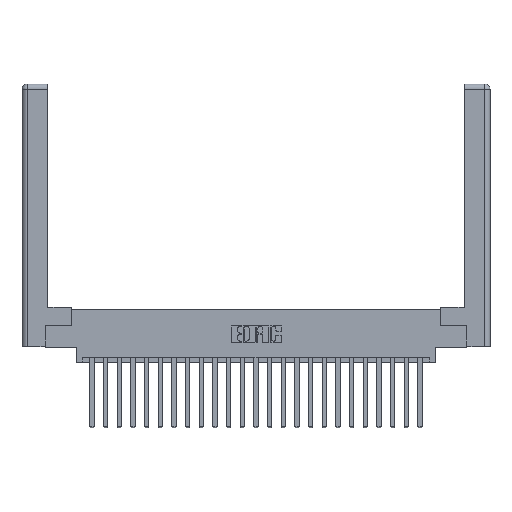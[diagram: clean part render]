
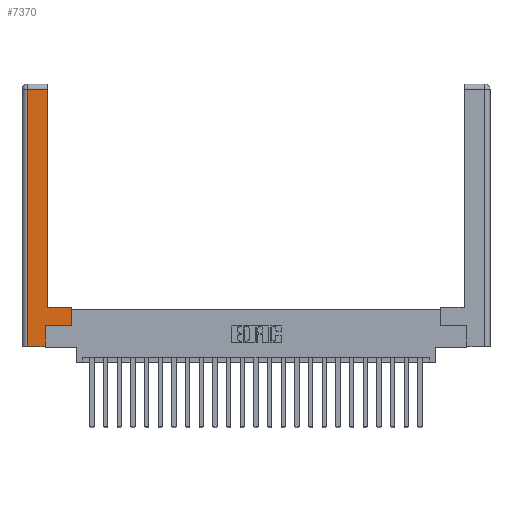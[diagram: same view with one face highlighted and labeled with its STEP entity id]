
A CAD part, top view. The second image highlights one B-rep face of the part: STEP entity #7370.
In plain terms, the highlighted planar face has unit normal (0, 0, 1).
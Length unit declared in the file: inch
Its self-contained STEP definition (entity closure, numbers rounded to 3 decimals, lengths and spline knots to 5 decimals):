
#581 = VECTOR ( 'NONE', #10612, 39.37008 ) ;
#743 = DIRECTION ( 'NONE',  ( 0., 0., -1. ) ) ;
#1216 = DIRECTION ( 'NONE',  ( 0., 1., 0. ) ) ;
#1859 = CARTESIAN_POINT ( 'NONE',  ( 0.295, 3., 0. ) ) ;
#2263 = LINE ( 'NONE', #6766, #19769 ) ;
#3188 = CARTESIAN_POINT ( 'NONE',  ( 0.0615, 2.94, 0. ) ) ;
#3585 = EDGE_CURVE ( 'NONE', #15018, #8057, #8193, .T. ) ;
#3625 = CARTESIAN_POINT ( 'NONE',  ( 0.265, 0.245, 0. ) ) ;
#3788 = CARTESIAN_POINT ( 'NONE',  ( 0.0615, 2.94, 0. ) ) ;
#4026 = EDGE_CURVE ( 'NONE', #7531, #15018, #9189, .T. ) ;
#4253 = LINE ( 'NONE', #15945, #17958 ) ;
#4887 = DIRECTION ( 'NONE',  ( 0., -1., 0. ) ) ;
#5621 = ORIENTED_EDGE ( 'NONE', *, *, #22635, .T. ) ;
#5629 = DIRECTION ( 'NONE',  ( 0., 1., 0. ) ) ;
#6648 = CARTESIAN_POINT ( 'NONE',  ( 0.565, 0.45, 0. ) ) ;
#6702 = VECTOR ( 'NONE', #11652, 39.37008 ) ;
#6766 = CARTESIAN_POINT ( 'NONE',  ( 0.0615, 0., 0. ) ) ;
#7274 = ORIENTED_EDGE ( 'NONE', *, *, #9608, .T. ) ;
#7370 = ADVANCED_FACE ( 'NONE', ( #11350 ), #13648, .F. ) ;
#7531 = VERTEX_POINT ( 'NONE', #12758 ) ;
#7633 = EDGE_CURVE ( 'NONE', #8057, #8959, #2263, .T. ) ;
#7858 = VERTEX_POINT ( 'NONE', #6648 ) ;
#8057 = VERTEX_POINT ( 'NONE', #3788 ) ;
#8137 = ORIENTED_EDGE ( 'NONE', *, *, #10321, .T. ) ;
#8193 = LINE ( 'NONE', #3188, #17519 ) ;
#8214 = CARTESIAN_POINT ( 'NONE',  ( 0.265, 0.245, 0. ) ) ;
#8261 = ORIENTED_EDGE ( 'NONE', *, *, #21714, .T. ) ;
#8896 = CARTESIAN_POINT ( 'NONE',  ( 0.265, 0., 0. ) ) ;
#8959 = VERTEX_POINT ( 'NONE', #15193 ) ;
#9189 = LINE ( 'NONE', #1859, #17067 ) ;
#9245 = VECTOR ( 'NONE', #22828, 39.37008 ) ;
#9492 = CARTESIAN_POINT ( 'NONE',  ( 0.565, 0.245, 0. ) ) ;
#9608 = EDGE_CURVE ( 'NONE', #8959, #12334, #4253, .T. ) ;
#10225 = DIRECTION ( 'NONE',  ( -1., 0., 0. ) ) ;
#10317 = EDGE_CURVE ( 'NONE', #19645, #7858, #21887, .T. ) ;
#10321 = EDGE_CURVE ( 'NONE', #14844, #19645, #12874, .T. ) ;
#10612 = DIRECTION ( 'NONE',  ( 1., 0., 0. ) ) ;
#10776 = DIRECTION ( 'NONE',  ( -1., 0., 0. ) ) ;
#10797 = ORIENTED_EDGE ( 'NONE', *, *, #4026, .T. ) ;
#11350 = FACE_OUTER_BOUND ( 'NONE', #13026, .T. ) ;
#11652 = DIRECTION ( 'NONE',  ( -1., 0., 0. ) ) ;
#11684 = LINE ( 'NONE', #22889, #6702 ) ;
#12209 = AXIS2_PLACEMENT_3D ( 'NONE', #13808, #743, #10225 ) ;
#12334 = VERTEX_POINT ( 'NONE', #8896 ) ;
#12758 = CARTESIAN_POINT ( 'NONE',  ( 0.295, 0.45, 0. ) ) ;
#12874 = LINE ( 'NONE', #15972, #581 ) ;
#13026 = EDGE_LOOP ( 'NONE', ( #10797, #18101, #19709, #7274, #8261, #8137, #15227, #5621 ) ) ;
#13648 = PLANE ( 'NONE',  #12209 ) ;
#13808 = CARTESIAN_POINT ( 'NONE',  ( 0., 0., 0. ) ) ;
#14000 = DIRECTION ( 'NONE',  ( 1., 0., 0. ) ) ;
#14189 = LINE ( 'NONE', #8214, #9245 ) ;
#14296 = VECTOR ( 'NONE', #1216, 39.37008 ) ;
#14844 = VERTEX_POINT ( 'NONE', #3625 ) ;
#15018 = VERTEX_POINT ( 'NONE', #17613 ) ;
#15193 = CARTESIAN_POINT ( 'NONE',  ( 0.0615, 0., 0. ) ) ;
#15227 = ORIENTED_EDGE ( 'NONE', *, *, #10317, .T. ) ;
#15945 = CARTESIAN_POINT ( 'NONE',  ( 0.265, 0., 0. ) ) ;
#15972 = CARTESIAN_POINT ( 'NONE',  ( 0.565, 0.245, 0. ) ) ;
#17067 = VECTOR ( 'NONE', #5629, 39.37008 ) ;
#17519 = VECTOR ( 'NONE', #10776, 39.37008 ) ;
#17613 = CARTESIAN_POINT ( 'NONE',  ( 0.295, 2.94, 0. ) ) ;
#17958 = VECTOR ( 'NONE', #14000, 39.37008 ) ;
#18101 = ORIENTED_EDGE ( 'NONE', *, *, #3585, .T. ) ;
#19645 = VERTEX_POINT ( 'NONE', #9492 ) ;
#19709 = ORIENTED_EDGE ( 'NONE', *, *, #7633, .T. ) ;
#19769 = VECTOR ( 'NONE', #4887, 39.37008 ) ;
#21714 = EDGE_CURVE ( 'NONE', #12334, #14844, #14189, .T. ) ;
#21866 = CARTESIAN_POINT ( 'NONE',  ( 0.565, 0.45, 0. ) ) ;
#21887 = LINE ( 'NONE', #21866, #14296 ) ;
#22635 = EDGE_CURVE ( 'NONE', #7858, #7531, #11684, .T. ) ;
#22828 = DIRECTION ( 'NONE',  ( 0., 1., 0. ) ) ;
#22889 = CARTESIAN_POINT ( 'NONE',  ( 0.295, 0.45, 0. ) ) ;
